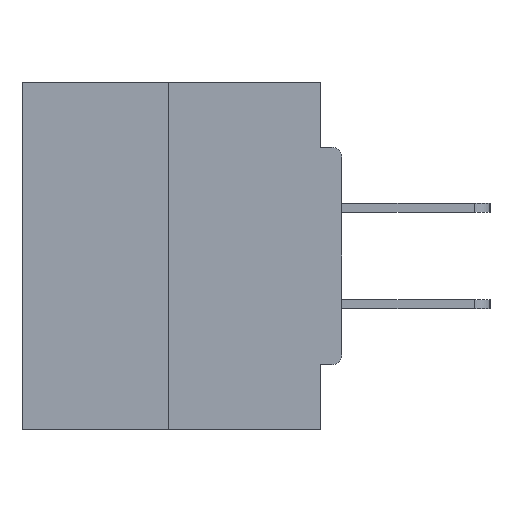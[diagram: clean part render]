
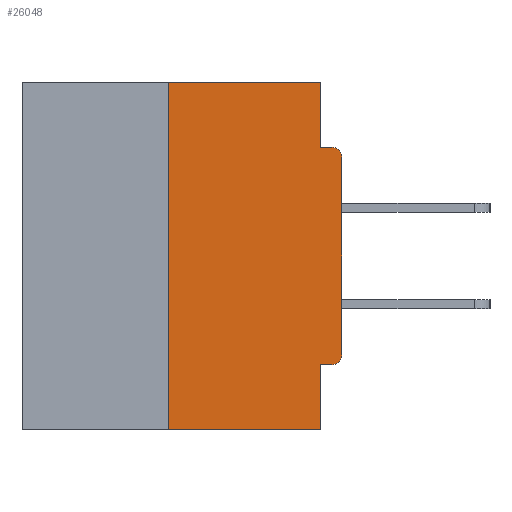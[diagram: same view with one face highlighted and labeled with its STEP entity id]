
A CAD part, left-side view. The second image highlights one B-rep face of the part: STEP entity #26048.
In plain terms, the highlighted planar face has unit normal (-1, 0, 0).
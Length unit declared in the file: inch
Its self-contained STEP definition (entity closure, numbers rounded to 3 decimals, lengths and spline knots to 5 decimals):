
#175 = EDGE_CURVE ( 'NONE', #21337, #5408, #11854, .T. ) ;
#281 = EDGE_CURVE ( 'NONE', #298, #20931, #5358, .T. ) ;
#298 = VERTEX_POINT ( 'NONE', #20758 ) ;
#363 = DIRECTION ( 'NONE',  ( 1., 0., 0. ) ) ;
#372 = LINE ( 'NONE', #32938, #4254 ) ;
#541 = VERTEX_POINT ( 'NONE', #23144 ) ;
#724 = ORIENTED_EDGE ( 'NONE', *, *, #2194, .T. ) ;
#1195 = CARTESIAN_POINT ( 'NONE',  ( 0., 0.015, -0.3915 ) ) ;
#1551 = CARTESIAN_POINT ( 'NONE',  ( 0., 0.46, 0. ) ) ;
#1639 = VECTOR ( 'NONE', #26833, 39.37008 ) ;
#1785 = CARTESIAN_POINT ( 'NONE',  ( 0., 0.031, -0.4065 ) ) ;
#2194 = EDGE_CURVE ( 'NONE', #12661, #541, #9562, .T. ) ;
#2374 = CARTESIAN_POINT ( 'NONE',  ( 0., 0.25, 0. ) ) ;
#2440 = AXIS2_PLACEMENT_3D ( 'NONE', #1195, #34826, #15247 ) ;
#2520 = LINE ( 'NONE', #7371, #1639 ) ;
#2795 = ORIENTED_EDGE ( 'NONE', *, *, #14066, .T. ) ;
#3212 = ORIENTED_EDGE ( 'NONE', *, *, #24462, .T. ) ;
#3279 = CARTESIAN_POINT ( 'NONE',  ( 0., 0., -0.3915 ) ) ;
#4028 = ORIENTED_EDGE ( 'NONE', *, *, #4457, .F. ) ;
#4254 = VECTOR ( 'NONE', #10911, 39.37008 ) ;
#4341 = CARTESIAN_POINT ( 'NONE',  ( 0., 0.031, 0. ) ) ;
#4347 = FACE_OUTER_BOUND ( 'NONE', #30077, .T. ) ;
#4457 = EDGE_CURVE ( 'NONE', #30588, #541, #2520, .T. ) ;
#5351 = LINE ( 'NONE', #4341, #25777 ) ;
#5358 = LINE ( 'NONE', #1551, #23191 ) ;
#5364 = CARTESIAN_POINT ( 'NONE',  ( 0., 0.031, 0. ) ) ;
#5408 = VERTEX_POINT ( 'NONE', #3279 ) ;
#5731 = CARTESIAN_POINT ( 'NONE',  ( 0., 0., -0.1085 ) ) ;
#5750 = AXIS2_PLACEMENT_3D ( 'NONE', #21809, #35760, #19138 ) ;
#7303 = VECTOR ( 'NONE', #8050, 39.37008 ) ;
#7371 = CARTESIAN_POINT ( 'NONE',  ( 0., 0.031, -0.5 ) ) ;
#8050 = DIRECTION ( 'NONE',  ( 0., 0., 1. ) ) ;
#8808 = ORIENTED_EDGE ( 'NONE', *, *, #26686, .F. ) ;
#9562 = LINE ( 'NONE', #9568, #26120 ) ;
#9568 = CARTESIAN_POINT ( 'NONE',  ( 0., 0.46, -0.5 ) ) ;
#10233 = VERTEX_POINT ( 'NONE', #32025 ) ;
#10521 = VECTOR ( 'NONE', #18855, 39.37008 ) ;
#10911 = DIRECTION ( 'NONE',  ( 0., -1., 0. ) ) ;
#11028 = EDGE_CURVE ( 'NONE', #21337, #30588, #17953, .T. ) ;
#11854 = CIRCLE ( 'NONE', #2440, 0.015 ) ;
#12661 = VERTEX_POINT ( 'NONE', #15957 ) ;
#14066 = EDGE_CURVE ( 'NONE', #5408, #21077, #30755, .T. ) ;
#15047 = DIRECTION ( 'NONE',  ( 0., -1., 0. ) ) ;
#15102 = CARTESIAN_POINT ( 'NONE',  ( 0., 0., 0. ) ) ;
#15247 = DIRECTION ( 'NONE',  ( 0., 0., -1. ) ) ;
#15957 = CARTESIAN_POINT ( 'NONE',  ( 0., 0.25, -0.5 ) ) ;
#16640 = ORIENTED_EDGE ( 'NONE', *, *, #27185, .F. ) ;
#17567 = PLANE ( 'NONE',  #26286 ) ;
#17762 = LINE ( 'NONE', #2374, #7303 ) ;
#17953 = LINE ( 'NONE', #21034, #10521 ) ;
#18855 = DIRECTION ( 'NONE',  ( 0., 1., 0. ) ) ;
#19138 = DIRECTION ( 'NONE',  ( 0., 0., -1. ) ) ;
#20758 = CARTESIAN_POINT ( 'NONE',  ( 0., 0.25, 0. ) ) ;
#20871 = DIRECTION ( 'NONE',  ( 0., -1., 0. ) ) ;
#20931 = VERTEX_POINT ( 'NONE', #5364 ) ;
#21034 = CARTESIAN_POINT ( 'NONE',  ( 0., 0., -0.4065 ) ) ;
#21077 = VERTEX_POINT ( 'NONE', #5731 ) ;
#21337 = VERTEX_POINT ( 'NONE', #32188 ) ;
#21809 = CARTESIAN_POINT ( 'NONE',  ( 0., 0.015, -0.1085 ) ) ;
#21997 = CARTESIAN_POINT ( 'NONE',  ( 0., 0.015, -0.0935 ) ) ;
#23037 = ORIENTED_EDGE ( 'NONE', *, *, #281, .F. ) ;
#23144 = CARTESIAN_POINT ( 'NONE',  ( 0., 0.031, -0.5 ) ) ;
#23191 = VECTOR ( 'NONE', #20871, 39.37008 ) ;
#23367 = VECTOR ( 'NONE', #29105, 39.37008 ) ;
#24292 = EDGE_CURVE ( 'NONE', #20931, #10233, #5351, .T. ) ;
#24462 = EDGE_CURVE ( 'NONE', #21077, #25618, #27956, .T. ) ;
#25618 = VERTEX_POINT ( 'NONE', #21997 ) ;
#25777 = VECTOR ( 'NONE', #31927, 39.37008 ) ;
#26048 = ADVANCED_FACE ( 'NONE', ( #4347 ), #17567, .F. ) ;
#26120 = VECTOR ( 'NONE', #15047, 39.37008 ) ;
#26286 = AXIS2_PLACEMENT_3D ( 'NONE', #34488, #363, #28784 ) ;
#26686 = EDGE_CURVE ( 'NONE', #12661, #298, #17762, .T. ) ;
#26833 = DIRECTION ( 'NONE',  ( 0., 0., -1. ) ) ;
#27185 = EDGE_CURVE ( 'NONE', #10233, #25618, #372, .T. ) ;
#27956 = CIRCLE ( 'NONE', #5750, 0.015 ) ;
#28657 = ORIENTED_EDGE ( 'NONE', *, *, #175, .T. ) ;
#28784 = DIRECTION ( 'NONE',  ( 0., 0., -1. ) ) ;
#29105 = DIRECTION ( 'NONE',  ( 0., 0., 1. ) ) ;
#29128 = ORIENTED_EDGE ( 'NONE', *, *, #11028, .F. ) ;
#30077 = EDGE_LOOP ( 'NONE', ( #23037, #8808, #724, #4028, #29128, #28657, #2795, #3212, #16640, #33550 ) ) ;
#30588 = VERTEX_POINT ( 'NONE', #1785 ) ;
#30755 = LINE ( 'NONE', #15102, #23367 ) ;
#31927 = DIRECTION ( 'NONE',  ( 0., 0., -1. ) ) ;
#32025 = CARTESIAN_POINT ( 'NONE',  ( 0., 0.031, -0.0935 ) ) ;
#32188 = CARTESIAN_POINT ( 'NONE',  ( 0., 0.015, -0.4065 ) ) ;
#32938 = CARTESIAN_POINT ( 'NONE',  ( 0., 0., -0.0935 ) ) ;
#33550 = ORIENTED_EDGE ( 'NONE', *, *, #24292, .F. ) ;
#34488 = CARTESIAN_POINT ( 'NONE',  ( 0., 0.46, 0. ) ) ;
#34826 = DIRECTION ( 'NONE',  ( -1., 0., 0. ) ) ;
#35760 = DIRECTION ( 'NONE',  ( -1., 0., 0. ) ) ;
